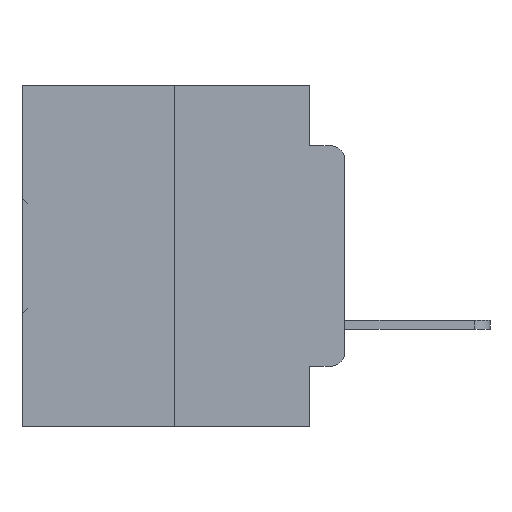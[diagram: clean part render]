
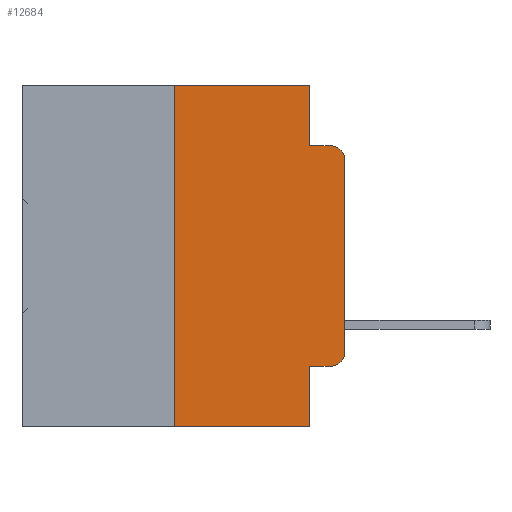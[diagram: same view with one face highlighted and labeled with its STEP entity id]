
A CAD part, left-side view. The second image highlights one B-rep face of the part: STEP entity #12684.
In plain terms, the highlighted planar face has unit normal (-1, 0, 0).
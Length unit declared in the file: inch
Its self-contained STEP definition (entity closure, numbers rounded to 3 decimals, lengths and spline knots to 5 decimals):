
#210 = CARTESIAN_POINT ( 'NONE',  ( 0., 0.051, -0.4115 ) ) ;
#746 = VECTOR ( 'NONE', #11574, 39.37008 ) ;
#918 = CARTESIAN_POINT ( 'NONE',  ( 0., 0.25, -0.5 ) ) ;
#927 = ORIENTED_EDGE ( 'NONE', *, *, #20705, .T. ) ;
#968 = CARTESIAN_POINT ( 'NONE',  ( 0., 0.051, -0.4115 ) ) ;
#1190 = CARTESIAN_POINT ( 'NONE',  ( 0., 0.473, 0. ) ) ;
#1200 = EDGE_CURVE ( 'NONE', #19179, #25122, #28637, .T. ) ;
#1489 = LINE ( 'NONE', #968, #15626 ) ;
#1839 = CARTESIAN_POINT ( 'NONE',  ( 0., 0.051, 0. ) ) ;
#2231 = ORIENTED_EDGE ( 'NONE', *, *, #20643, .T. ) ;
#4317 = CARTESIAN_POINT ( 'NONE',  ( 0., 0.051, 0. ) ) ;
#4710 = DIRECTION ( 'NONE',  ( 0., 0., -1. ) ) ;
#4729 = CARTESIAN_POINT ( 'NONE',  ( 0., 0.02, -0.3915 ) ) ;
#5292 = DIRECTION ( 'NONE',  ( 0., -1., 0. ) ) ;
#5474 = EDGE_CURVE ( 'NONE', #7595, #19659, #9760, .T. ) ;
#5873 = CARTESIAN_POINT ( 'NONE',  ( 0., 0., -0.3915 ) ) ;
#6031 = LINE ( 'NONE', #4317, #33727 ) ;
#6690 = ORIENTED_EDGE ( 'NONE', *, *, #10987, .F. ) ;
#7595 = VERTEX_POINT ( 'NONE', #20338 ) ;
#7605 = DIRECTION ( 'NONE',  ( 0., 0., -1. ) ) ;
#8206 = VECTOR ( 'NONE', #4710, 39.37008 ) ;
#9347 = LINE ( 'NONE', #21316, #29996 ) ;
#9760 = LINE ( 'NONE', #17061, #16249 ) ;
#10101 = AXIS2_PLACEMENT_3D ( 'NONE', #23431, #23398, #23517 ) ;
#10293 = ORIENTED_EDGE ( 'NONE', *, *, #33394, .T. ) ;
#10656 = EDGE_CURVE ( 'NONE', #20051, #7595, #15767, .T. ) ;
#10987 = EDGE_CURVE ( 'NONE', #26864, #14865, #6031, .T. ) ;
#11100 = VERTEX_POINT ( 'NONE', #13367 ) ;
#11546 = EDGE_LOOP ( 'NONE', ( #2231, #24394, #31245, #18893, #32760, #20641, #27594, #6690, #927, #10293 ) ) ;
#11574 = DIRECTION ( 'NONE',  ( 0., 0., 1. ) ) ;
#12442 = DIRECTION ( 'NONE',  ( 0., -1., 0. ) ) ;
#12617 = LINE ( 'NONE', #21966, #33613 ) ;
#12658 = DIRECTION ( 'NONE',  ( 1., 0., 0. ) ) ;
#12684 = ADVANCED_FACE ( 'NONE', ( #18482 ), #26096, .F. ) ;
#13279 = CARTESIAN_POINT ( 'NONE',  ( 0., 0.02, -0.0885 ) ) ;
#13367 = CARTESIAN_POINT ( 'NONE',  ( 0., 0.051, -0.0885 ) ) ;
#14865 = VERTEX_POINT ( 'NONE', #19942 ) ;
#15326 = VERTEX_POINT ( 'NONE', #5873 ) ;
#15626 = VECTOR ( 'NONE', #12442, 39.37008 ) ;
#15767 = LINE ( 'NONE', #27674, #746 ) ;
#15984 = CARTESIAN_POINT ( 'NONE',  ( 0., 0.051, 0. ) ) ;
#16249 = VECTOR ( 'NONE', #16611, 39.37008 ) ;
#16299 = CIRCLE ( 'NONE', #31334, 0.02 ) ;
#16433 = CARTESIAN_POINT ( 'NONE',  ( 0., 0.02, -0.4115 ) ) ;
#16611 = DIRECTION ( 'NONE',  ( 0., -1., 0. ) ) ;
#16918 = AXIS2_PLACEMENT_3D ( 'NONE', #1190, #12658, #31256 ) ;
#17061 = CARTESIAN_POINT ( 'NONE',  ( 0., 0.473, 0. ) ) ;
#17354 = LINE ( 'NONE', #1839, #8206 ) ;
#18482 = FACE_OUTER_BOUND ( 'NONE', #11546, .T. ) ;
#18893 = ORIENTED_EDGE ( 'NONE', *, *, #20371, .F. ) ;
#19179 = VERTEX_POINT ( 'NONE', #32447 ) ;
#19659 = VERTEX_POINT ( 'NONE', #15984 ) ;
#19942 = CARTESIAN_POINT ( 'NONE',  ( 0., 0.051, -0.5 ) ) ;
#20051 = VERTEX_POINT ( 'NONE', #918 ) ;
#20338 = CARTESIAN_POINT ( 'NONE',  ( 0., 0.25, 0. ) ) ;
#20371 = EDGE_CURVE ( 'NONE', #19659, #11100, #17354, .T. ) ;
#20641 = ORIENTED_EDGE ( 'NONE', *, *, #10656, .F. ) ;
#20643 = EDGE_CURVE ( 'NONE', #15326, #19179, #33637, .T. ) ;
#20705 = EDGE_CURVE ( 'NONE', #26864, #20966, #1489, .T. ) ;
#20945 = EDGE_CURVE ( 'NONE', #20051, #14865, #12617, .T. ) ;
#20966 = VERTEX_POINT ( 'NONE', #16433 ) ;
#21316 = CARTESIAN_POINT ( 'NONE',  ( 0., 0.051, -0.0885 ) ) ;
#21966 = CARTESIAN_POINT ( 'NONE',  ( 0., 0.473, -0.5 ) ) ;
#22801 = CARTESIAN_POINT ( 'NONE',  ( 0., 0., 0. ) ) ;
#23398 = DIRECTION ( 'NONE',  ( -1., 0., 0. ) ) ;
#23431 = CARTESIAN_POINT ( 'NONE',  ( 0., 0.02, -0.1085 ) ) ;
#23517 = DIRECTION ( 'NONE',  ( 0., 0., -1. ) ) ;
#24109 = DIRECTION ( 'NONE',  ( -1., 0., 0. ) ) ;
#24394 = ORIENTED_EDGE ( 'NONE', *, *, #1200, .T. ) ;
#25122 = VERTEX_POINT ( 'NONE', #13279 ) ;
#25450 = DIRECTION ( 'NONE',  ( 0., 0., 1. ) ) ;
#26096 = PLANE ( 'NONE',  #16918 ) ;
#26337 = DIRECTION ( 'NONE',  ( 0., 0., -1. ) ) ;
#26864 = VERTEX_POINT ( 'NONE', #210 ) ;
#27594 = ORIENTED_EDGE ( 'NONE', *, *, #20945, .T. ) ;
#27674 = CARTESIAN_POINT ( 'NONE',  ( 0., 0.25, 0. ) ) ;
#28112 = EDGE_CURVE ( 'NONE', #11100, #25122, #9347, .T. ) ;
#28637 = CIRCLE ( 'NONE', #10101, 0.02 ) ;
#29996 = VECTOR ( 'NONE', #34166, 39.37008 ) ;
#31245 = ORIENTED_EDGE ( 'NONE', *, *, #28112, .F. ) ;
#31256 = DIRECTION ( 'NONE',  ( 0., 0., -1. ) ) ;
#31334 = AXIS2_PLACEMENT_3D ( 'NONE', #4729, #24109, #7605 ) ;
#32447 = CARTESIAN_POINT ( 'NONE',  ( 0., 0., -0.1085 ) ) ;
#32760 = ORIENTED_EDGE ( 'NONE', *, *, #5474, .F. ) ;
#32876 = VECTOR ( 'NONE', #25450, 39.37008 ) ;
#33394 = EDGE_CURVE ( 'NONE', #20966, #15326, #16299, .T. ) ;
#33613 = VECTOR ( 'NONE', #5292, 39.37008 ) ;
#33637 = LINE ( 'NONE', #22801, #32876 ) ;
#33727 = VECTOR ( 'NONE', #26337, 39.37008 ) ;
#34166 = DIRECTION ( 'NONE',  ( 0., -1., 0. ) ) ;
